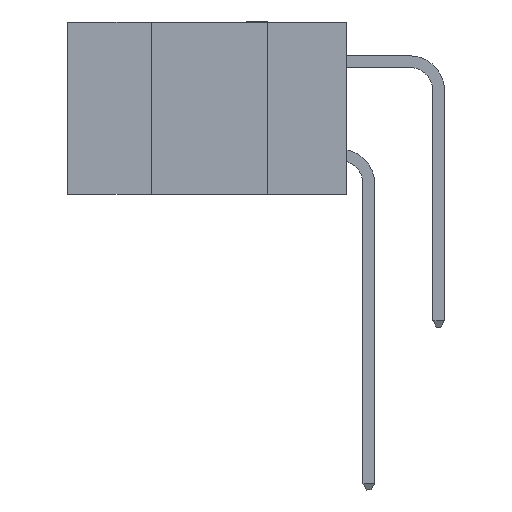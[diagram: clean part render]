
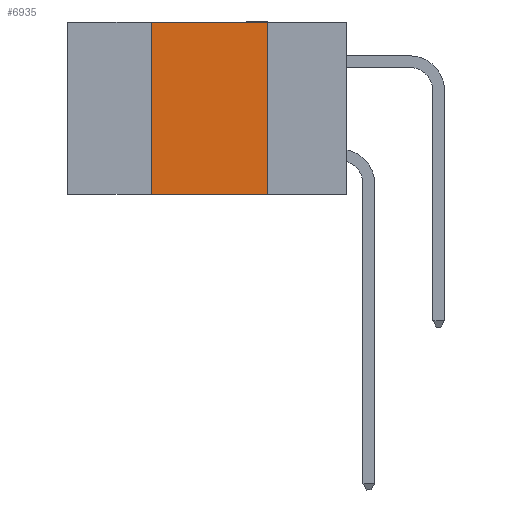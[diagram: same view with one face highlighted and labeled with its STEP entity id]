
A CAD part, left-side view. The second image highlights one B-rep face of the part: STEP entity #6935.
In plain terms, the highlighted planar face has unit normal (-1, 0, 0).
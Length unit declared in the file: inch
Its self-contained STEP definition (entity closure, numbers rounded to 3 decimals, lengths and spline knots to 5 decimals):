
#708 = VERTEX_POINT ( 'NONE', #11539 ) ;
#724 = ORIENTED_EDGE ( 'NONE', *, *, #3820, .T. ) ;
#1213 = DIRECTION ( 'NONE',  ( 0., 0., -1. ) ) ;
#1267 = CARTESIAN_POINT ( 'NONE',  ( 0., 0.42, 0. ) ) ;
#1538 = VECTOR ( 'NONE', #19330, 39.37008 ) ;
#1578 = DIRECTION ( 'NONE',  ( 0., -1., 0. ) ) ;
#3791 = VERTEX_POINT ( 'NONE', #18293 ) ;
#3820 = EDGE_CURVE ( 'NONE', #15980, #3791, #17208, .T. ) ;
#4847 = EDGE_CURVE ( 'NONE', #15980, #708, #18278, .T. ) ;
#5473 = VERTEX_POINT ( 'NONE', #11455 ) ;
#6648 = VECTOR ( 'NONE', #12129, 39.37008 ) ;
#6734 = VECTOR ( 'NONE', #9837, 39.37008 ) ;
#6935 = ADVANCED_FACE ( 'NONE', ( #12684 ), #8956, .F. ) ;
#6997 = ORIENTED_EDGE ( 'NONE', *, *, #10063, .F. ) ;
#7227 = CARTESIAN_POINT ( 'NONE',  ( 0., 0.6, 0. ) ) ;
#7247 = CARTESIAN_POINT ( 'NONE',  ( 0., 0.17, 0. ) ) ;
#8672 = VECTOR ( 'NONE', #1578, 39.37008 ) ;
#8956 = PLANE ( 'NONE',  #14813 ) ;
#9310 = EDGE_CURVE ( 'NONE', #708, #5473, #10436, .T. ) ;
#9837 = DIRECTION ( 'NONE',  ( 0., -1., 0. ) ) ;
#10063 = EDGE_CURVE ( 'NONE', #5473, #3791, #13922, .T. ) ;
#10436 = LINE ( 'NONE', #18777, #6734 ) ;
#10525 = DIRECTION ( 'NONE',  ( 1., 0., 0. ) ) ;
#11455 = CARTESIAN_POINT ( 'NONE',  ( 0., 0.17, 0. ) ) ;
#11539 = CARTESIAN_POINT ( 'NONE',  ( 0., 0.42, 0. ) ) ;
#11652 = ORIENTED_EDGE ( 'NONE', *, *, #9310, .F. ) ;
#12129 = DIRECTION ( 'NONE',  ( 0., 0., 1. ) ) ;
#12684 = FACE_OUTER_BOUND ( 'NONE', #13253, .T. ) ;
#13253 = EDGE_LOOP ( 'NONE', ( #6997, #11652, #16141, #724 ) ) ;
#13922 = LINE ( 'NONE', #7247, #1538 ) ;
#14813 = AXIS2_PLACEMENT_3D ( 'NONE', #7227, #10525, #1213 ) ;
#15980 = VERTEX_POINT ( 'NONE', #19283 ) ;
#16141 = ORIENTED_EDGE ( 'NONE', *, *, #4847, .F. ) ;
#16917 = CARTESIAN_POINT ( 'NONE',  ( 0., 0.6, -0.37 ) ) ;
#17208 = LINE ( 'NONE', #16917, #8672 ) ;
#18278 = LINE ( 'NONE', #1267, #6648 ) ;
#18293 = CARTESIAN_POINT ( 'NONE',  ( 0., 0.17, -0.37 ) ) ;
#18777 = CARTESIAN_POINT ( 'NONE',  ( 0., 0.6, 0. ) ) ;
#19283 = CARTESIAN_POINT ( 'NONE',  ( 0., 0.42, -0.37 ) ) ;
#19330 = DIRECTION ( 'NONE',  ( 0., 0., -1. ) ) ;
